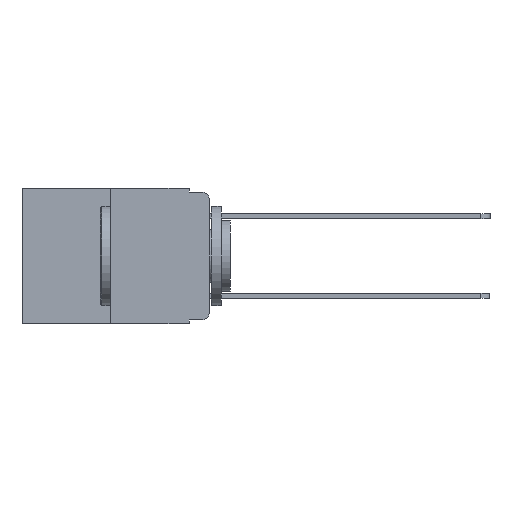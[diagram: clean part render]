
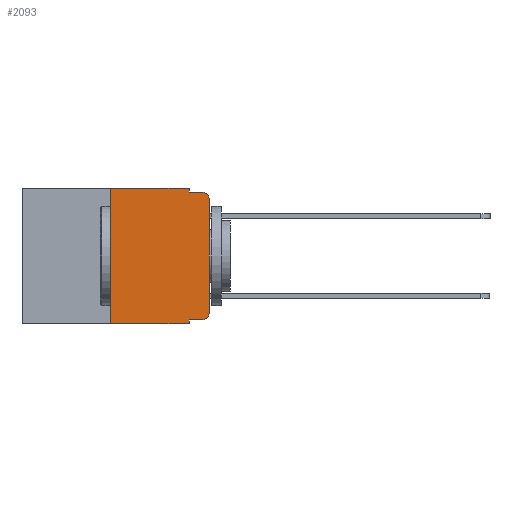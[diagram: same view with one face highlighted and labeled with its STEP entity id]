
A CAD part, left-side view. The second image highlights one B-rep face of the part: STEP entity #2093.
In plain terms, the highlighted planar face has unit normal (-1, 0, 0).
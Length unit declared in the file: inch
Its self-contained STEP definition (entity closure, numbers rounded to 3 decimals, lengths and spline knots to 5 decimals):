
#73 = CARTESIAN_POINT ( 'NONE',  ( 0., 0.473, -0.343 ) ) ;
#316 = AXIS2_PLACEMENT_3D ( 'NONE', #1185, #21147, #20936 ) ;
#490 = AXIS2_PLACEMENT_3D ( 'NONE', #11966, #26073, #14046 ) ;
#908 = EDGE_LOOP ( 'NONE', ( #15232, #14864, #12843, #20525, #14319, #13873, #13505, #11962, #11264, #10974 ) ) ;
#1092 = VECTOR ( 'NONE', #23062, 39.37008 ) ;
#1185 = CARTESIAN_POINT ( 'NONE',  ( 0., 0.473, 0. ) ) ;
#1762 = EDGE_CURVE ( 'NONE', #11770, #24736, #12631, .T. ) ;
#2093 = ADVANCED_FACE ( 'NONE', ( #21206 ), #23809, .F. ) ;
#2964 = VERTEX_POINT ( 'NONE', #17570 ) ;
#3038 = LINE ( 'NONE', #23839, #24066 ) ;
#3051 = DIRECTION ( 'NONE',  ( 0., 0., -1. ) ) ;
#3666 = CARTESIAN_POINT ( 'NONE',  ( 0., 0.02, -0.333 ) ) ;
#4085 = VERTEX_POINT ( 'NONE', #4134 ) ;
#4134 = CARTESIAN_POINT ( 'NONE',  ( 0., 0., -0.03 ) ) ;
#4237 = VECTOR ( 'NONE', #11326, 39.37008 ) ;
#5148 = CARTESIAN_POINT ( 'NONE',  ( 0., 0.25, 0. ) ) ;
#5177 = DIRECTION ( 'NONE',  ( 0., -1., 0. ) ) ;
#5638 = VECTOR ( 'NONE', #26352, 39.37008 ) ;
#6279 = CARTESIAN_POINT ( 'NONE',  ( 0., 0., 0. ) ) ;
#6485 = CARTESIAN_POINT ( 'NONE',  ( 0., 0.051, -0.01 ) ) ;
#6780 = CARTESIAN_POINT ( 'NONE',  ( 0., 0.051, 0. ) ) ;
#7188 = VECTOR ( 'NONE', #14593, 39.37008 ) ;
#7298 = DIRECTION ( 'NONE',  ( 0., 0., -1. ) ) ;
#7320 = EDGE_CURVE ( 'NONE', #23799, #11770, #3038, .T. ) ;
#7438 = CARTESIAN_POINT ( 'NONE',  ( 0., 0.02, -0.313 ) ) ;
#7685 = CARTESIAN_POINT ( 'NONE',  ( 0., 0.051, 0. ) ) ;
#7816 = VECTOR ( 'NONE', #10357, 39.37008 ) ;
#8094 = VERTEX_POINT ( 'NONE', #6485 ) ;
#9145 = CARTESIAN_POINT ( 'NONE',  ( 0., 0.051, 0. ) ) ;
#9649 = LINE ( 'NONE', #5148, #4237 ) ;
#10357 = DIRECTION ( 'NONE',  ( 0., 0., 1. ) ) ;
#10619 = VECTOR ( 'NONE', #3051, 39.37008 ) ;
#10974 = ORIENTED_EDGE ( 'NONE', *, *, #1762, .T. ) ;
#11264 = ORIENTED_EDGE ( 'NONE', *, *, #7320, .T. ) ;
#11326 = DIRECTION ( 'NONE',  ( 0., 0., 1. ) ) ;
#11455 = EDGE_CURVE ( 'NONE', #23799, #21416, #16077, .T. ) ;
#11729 = DIRECTION ( 'NONE',  ( 0., -1., 0. ) ) ;
#11770 = VERTEX_POINT ( 'NONE', #3666 ) ;
#11962 = ORIENTED_EDGE ( 'NONE', *, *, #11455, .F. ) ;
#11966 = CARTESIAN_POINT ( 'NONE',  ( 0., 0.02, -0.03 ) ) ;
#12376 = LINE ( 'NONE', #6780, #1092 ) ;
#12626 = LINE ( 'NONE', #73, #7188 ) ;
#12631 = CIRCLE ( 'NONE', #20656, 0.02 ) ;
#12843 = ORIENTED_EDGE ( 'NONE', *, *, #16410, .F. ) ;
#13505 = ORIENTED_EDGE ( 'NONE', *, *, #24046, .T. ) ;
#13873 = ORIENTED_EDGE ( 'NONE', *, *, #18276, .F. ) ;
#14046 = DIRECTION ( 'NONE',  ( 0., 0., -1. ) ) ;
#14279 = VERTEX_POINT ( 'NONE', #15255 ) ;
#14319 = ORIENTED_EDGE ( 'NONE', *, *, #22477, .F. ) ;
#14593 = DIRECTION ( 'NONE',  ( 0., -1., 0. ) ) ;
#14864 = ORIENTED_EDGE ( 'NONE', *, *, #22675, .T. ) ;
#15232 = ORIENTED_EDGE ( 'NONE', *, *, #24008, .T. ) ;
#15255 = CARTESIAN_POINT ( 'NONE',  ( 0., 0.25, 0. ) ) ;
#15893 = CARTESIAN_POINT ( 'NONE',  ( 0., 0., -0.313 ) ) ;
#16077 = LINE ( 'NONE', #9145, #10619 ) ;
#16410 = EDGE_CURVE ( 'NONE', #8094, #24963, #21891, .T. ) ;
#17254 = DIRECTION ( 'NONE',  ( -1., 0., 0. ) ) ;
#17570 = CARTESIAN_POINT ( 'NONE',  ( 0., 0.25, -0.343 ) ) ;
#18276 = EDGE_CURVE ( 'NONE', #2964, #14279, #9649, .T. ) ;
#19467 = CARTESIAN_POINT ( 'NONE',  ( 0., 0.473, 0. ) ) ;
#20034 = CIRCLE ( 'NONE', #490, 0.02 ) ;
#20525 = ORIENTED_EDGE ( 'NONE', *, *, #22332, .F. ) ;
#20656 = AXIS2_PLACEMENT_3D ( 'NONE', #7438, #17254, #7298 ) ;
#20658 = CARTESIAN_POINT ( 'NONE',  ( 0., 0.02, -0.01 ) ) ;
#20936 = DIRECTION ( 'NONE',  ( 0., 0., -1. ) ) ;
#21147 = DIRECTION ( 'NONE',  ( 1., 0., 0. ) ) ;
#21206 = FACE_OUTER_BOUND ( 'NONE', #908, .T. ) ;
#21416 = VERTEX_POINT ( 'NONE', #23474 ) ;
#21891 = LINE ( 'NONE', #24366, #5638 ) ;
#21948 = CARTESIAN_POINT ( 'NONE',  ( 0., 0.051, -0.333 ) ) ;
#22332 = EDGE_CURVE ( 'NONE', #25861, #8094, #12376, .T. ) ;
#22477 = EDGE_CURVE ( 'NONE', #14279, #25861, #24432, .T. ) ;
#22675 = EDGE_CURVE ( 'NONE', #4085, #24963, #20034, .T. ) ;
#23062 = DIRECTION ( 'NONE',  ( 0., 0., -1. ) ) ;
#23474 = CARTESIAN_POINT ( 'NONE',  ( 0., 0.051, -0.343 ) ) ;
#23799 = VERTEX_POINT ( 'NONE', #21948 ) ;
#23802 = VECTOR ( 'NONE', #5177, 39.37008 ) ;
#23809 = PLANE ( 'NONE',  #316 ) ;
#23839 = CARTESIAN_POINT ( 'NONE',  ( 0., 0.051, -0.333 ) ) ;
#24008 = EDGE_CURVE ( 'NONE', #24736, #4085, #24660, .T. ) ;
#24046 = EDGE_CURVE ( 'NONE', #2964, #21416, #12626, .T. ) ;
#24066 = VECTOR ( 'NONE', #11729, 39.37008 ) ;
#24366 = CARTESIAN_POINT ( 'NONE',  ( 0., 0.051, -0.01 ) ) ;
#24432 = LINE ( 'NONE', #19467, #23802 ) ;
#24660 = LINE ( 'NONE', #6279, #7816 ) ;
#24736 = VERTEX_POINT ( 'NONE', #15893 ) ;
#24963 = VERTEX_POINT ( 'NONE', #20658 ) ;
#25861 = VERTEX_POINT ( 'NONE', #7685 ) ;
#26073 = DIRECTION ( 'NONE',  ( -1., 0., 0. ) ) ;
#26352 = DIRECTION ( 'NONE',  ( 0., -1., 0. ) ) ;
